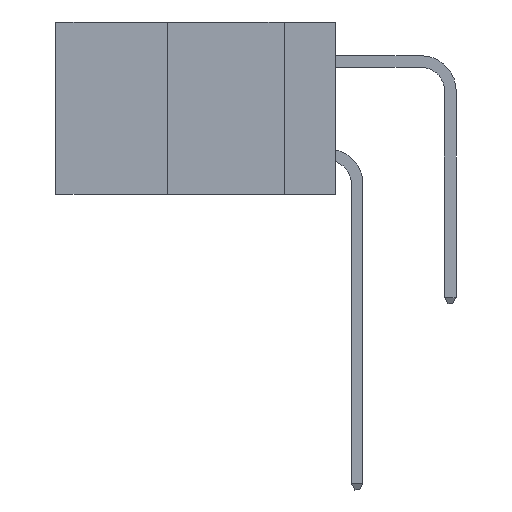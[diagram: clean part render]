
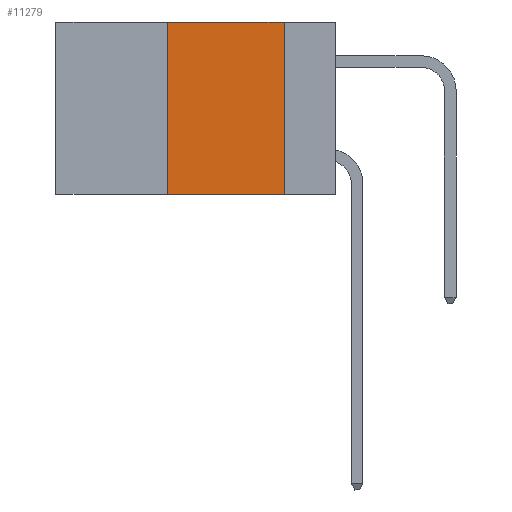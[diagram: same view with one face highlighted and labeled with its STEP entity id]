
A CAD part, left-side view. The second image highlights one B-rep face of the part: STEP entity #11279.
In plain terms, the highlighted planar face has unit normal (-1, 0, 0).
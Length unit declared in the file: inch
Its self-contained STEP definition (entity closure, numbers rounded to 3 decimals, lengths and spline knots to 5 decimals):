
#221 = VERTEX_POINT ( 'NONE', #1297 ) ;
#891 = DIRECTION ( 'NONE',  ( 1., 0., 0. ) ) ;
#1297 = CARTESIAN_POINT ( 'NONE',  ( 0., 0.11, 0. ) ) ;
#1483 = VECTOR ( 'NONE', #12262, 39.37008 ) ;
#2117 = ORIENTED_EDGE ( 'NONE', *, *, #8932, .F. ) ;
#2302 = DIRECTION ( 'NONE',  ( 0., 0., -1. ) ) ;
#2489 = CARTESIAN_POINT ( 'NONE',  ( 0., 0.6, -0.37 ) ) ;
#2921 = DIRECTION ( 'NONE',  ( 0., 0., 1. ) ) ;
#3119 = CARTESIAN_POINT ( 'NONE',  ( 0., 0.6, 0. ) ) ;
#3364 = EDGE_CURVE ( 'NONE', #6878, #11603, #6237, .T. ) ;
#3645 = CARTESIAN_POINT ( 'NONE',  ( 0., 0.11, 0. ) ) ;
#4261 = CARTESIAN_POINT ( 'NONE',  ( 0., 0.36, 0. ) ) ;
#4660 = ORIENTED_EDGE ( 'NONE', *, *, #7882, .F. ) ;
#5383 = VERTEX_POINT ( 'NONE', #6476 ) ;
#6237 = LINE ( 'NONE', #4261, #7213 ) ;
#6476 = CARTESIAN_POINT ( 'NONE',  ( 0., 0.11, -0.37 ) ) ;
#6603 = CARTESIAN_POINT ( 'NONE',  ( 0., 0.36, -0.37 ) ) ;
#6878 = VERTEX_POINT ( 'NONE', #6603 ) ;
#7213 = VECTOR ( 'NONE', #2921, 39.37008 ) ;
#7325 = EDGE_CURVE ( 'NONE', #6878, #5383, #12981, .T. ) ;
#7485 = CARTESIAN_POINT ( 'NONE',  ( 0., 0.6, 0. ) ) ;
#7882 = EDGE_CURVE ( 'NONE', #11603, #221, #7996, .T. ) ;
#7996 = LINE ( 'NONE', #7485, #1483 ) ;
#8244 = PLANE ( 'NONE',  #9206 ) ;
#8874 = ORIENTED_EDGE ( 'NONE', *, *, #3364, .F. ) ;
#8932 = EDGE_CURVE ( 'NONE', #221, #5383, #13491, .T. ) ;
#9183 = EDGE_LOOP ( 'NONE', ( #2117, #4660, #8874, #14967 ) ) ;
#9206 = AXIS2_PLACEMENT_3D ( 'NONE', #3119, #891, #9457 ) ;
#9457 = DIRECTION ( 'NONE',  ( 0., 0., -1. ) ) ;
#11279 = ADVANCED_FACE ( 'NONE', ( #13306 ), #8244, .F. ) ;
#11439 = VECTOR ( 'NONE', #12275, 39.37008 ) ;
#11603 = VERTEX_POINT ( 'NONE', #15325 ) ;
#12262 = DIRECTION ( 'NONE',  ( 0., -1., 0. ) ) ;
#12275 = DIRECTION ( 'NONE',  ( 0., -1., 0. ) ) ;
#12981 = LINE ( 'NONE', #2489, #11439 ) ;
#13306 = FACE_OUTER_BOUND ( 'NONE', #9183, .T. ) ;
#13491 = LINE ( 'NONE', #3645, #14426 ) ;
#14426 = VECTOR ( 'NONE', #2302, 39.37008 ) ;
#14967 = ORIENTED_EDGE ( 'NONE', *, *, #7325, .T. ) ;
#15325 = CARTESIAN_POINT ( 'NONE',  ( 0., 0.36, 0. ) ) ;
